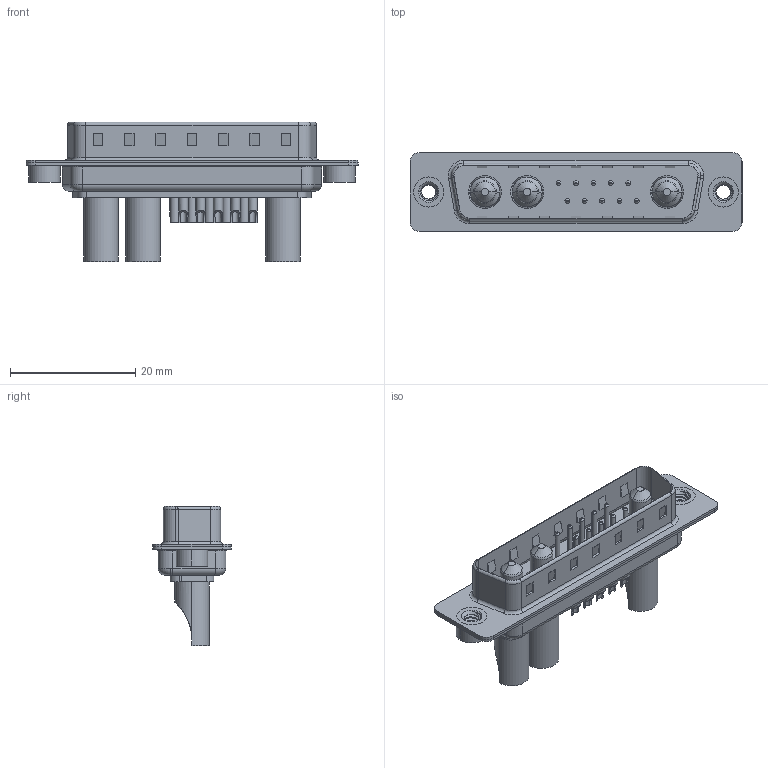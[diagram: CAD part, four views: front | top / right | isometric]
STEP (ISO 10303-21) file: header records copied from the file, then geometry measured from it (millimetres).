
FILE_DESCRIPTION (( 'STEP AP203' ), '1' );
FILE_NAME ('627-13W3222-4T2.STEP', '2019-05-26T12:18:30', ( '' ), ( '' ), 'SwSTEP 2.0', 'SolidWorks 2016', '' );
FILE_SCHEMA (( 'CONFIG_CONTROL_DESIGN' ));
Length unit declared in the file: millimetre
Products named in the file (8): 627Combo Shell Front_25 Contacts; 627Combo Threaded Rivet_2; Power Pin_40A SC; 627Combo Contact Row 1_22; 627Combo Contact Row 2_22; 627-13W3222-4T2; 627Combo Housing_13W3; 627Combo Shell Rear_25 Contacts
Assembly tree (18 placements, depth 2):
  627-13W3222-4T2
    627Combo Housing_13W3
    627Combo Shell Rear_25 Contacts
    627Combo Shell Front_25 Contacts
    627Combo Threaded Rivet_2  x2
    Power Pin_40A SC  x3
    627Combo Contact Row 1_22  x5
    627Combo Contact Row 2_22  x5
Bounding box: 53 x 12.6 x 22.3 mm (x, y, z)
Volume: 3060.3 mm3; surface area: 7248.4 mm2
Topology: 21 solids, 21 shells, 875 faces, 2085 edges, 1283 vertices
Faces by surface type: cylinder 357, plane 297, torus 156, cone 53, bspline 12
Entity records: 18531 total; most frequent: CARTESIAN_POINT 4399, DIRECTION 2864, ORIENTED_EDGE 2600, EDGE_CURVE 1300, AXIS2_PLACEMENT_3D 1089, VERTEX_POINT 821, VECTOR 686, LINE 686
